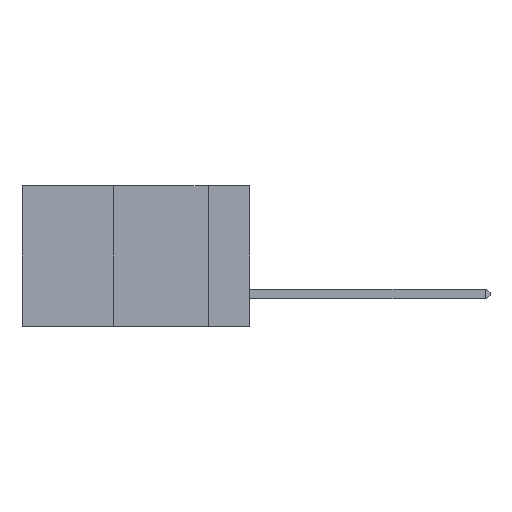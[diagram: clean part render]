
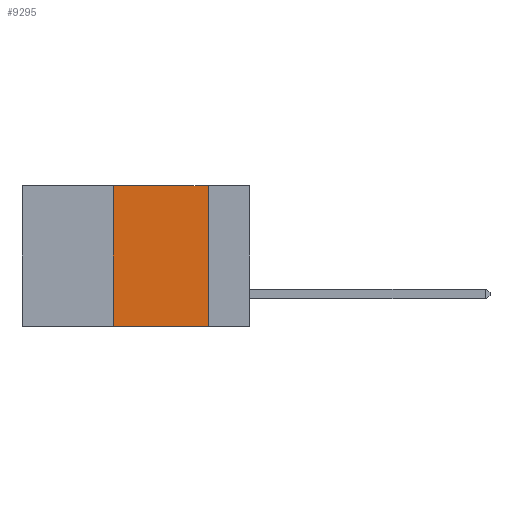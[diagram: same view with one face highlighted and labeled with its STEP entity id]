
A CAD part, left-side view. The second image highlights one B-rep face of the part: STEP entity #9295.
In plain terms, the highlighted planar face has unit normal (-1, 0, 0).
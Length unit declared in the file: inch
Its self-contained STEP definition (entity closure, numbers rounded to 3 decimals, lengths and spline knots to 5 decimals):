
#274 = ORIENTED_EDGE ( 'NONE', *, *, #9508, .F. ) ;
#290 = ORIENTED_EDGE ( 'NONE', *, *, #12163, .F. ) ;
#353 = ORIENTED_EDGE ( 'NONE', *, *, #3737, .F. ) ;
#403 = LINE ( 'NONE', #6212, #2656 ) ;
#404 = ORIENTED_EDGE ( 'NONE', *, *, #12074, .T. ) ;
#520 = LINE ( 'NONE', #2945, #10806 ) ;
#1215 = AXIS2_PLACEMENT_3D ( 'NONE', #3625, #4772, #11905 ) ;
#1304 = VERTEX_POINT ( 'NONE', #1729 ) ;
#1729 = CARTESIAN_POINT ( 'NONE',  ( 0., 0.36, -0.37 ) ) ;
#1730 = LINE ( 'NONE', #8205, #6918 ) ;
#2656 = VECTOR ( 'NONE', #5117, 39.37008 ) ;
#2933 = VECTOR ( 'NONE', #11274, 39.37008 ) ;
#2945 = CARTESIAN_POINT ( 'NONE',  ( 0., 0.36, 0. ) ) ;
#3074 = VERTEX_POINT ( 'NONE', #5282 ) ;
#3278 = LINE ( 'NONE', #10295, #2933 ) ;
#3625 = CARTESIAN_POINT ( 'NONE',  ( 0., 0.6, 0. ) ) ;
#3737 = EDGE_CURVE ( 'NONE', #1304, #3074, #520, .T. ) ;
#4772 = DIRECTION ( 'NONE',  ( 1., 0., 0. ) ) ;
#5117 = DIRECTION ( 'NONE',  ( 0., 0., -1. ) ) ;
#5282 = CARTESIAN_POINT ( 'NONE',  ( 0., 0.36, 0. ) ) ;
#6144 = DIRECTION ( 'NONE',  ( 0., -1., 0. ) ) ;
#6212 = CARTESIAN_POINT ( 'NONE',  ( 0., 0.11, 0. ) ) ;
#6918 = VECTOR ( 'NONE', #6144, 39.37008 ) ;
#7925 = CARTESIAN_POINT ( 'NONE',  ( 0., 0.11, 0. ) ) ;
#8205 = CARTESIAN_POINT ( 'NONE',  ( 0., 0.6, -0.37 ) ) ;
#9295 = ADVANCED_FACE ( 'NONE', ( #13478 ), #9951, .F. ) ;
#9508 = EDGE_CURVE ( 'NONE', #11434, #10222, #403, .T. ) ;
#9951 = PLANE ( 'NONE',  #1215 ) ;
#10222 = VERTEX_POINT ( 'NONE', #10843 ) ;
#10295 = CARTESIAN_POINT ( 'NONE',  ( 0., 0.6, 0. ) ) ;
#10358 = DIRECTION ( 'NONE',  ( 0., 0., 1. ) ) ;
#10806 = VECTOR ( 'NONE', #10358, 39.37008 ) ;
#10843 = CARTESIAN_POINT ( 'NONE',  ( 0., 0.11, -0.37 ) ) ;
#11274 = DIRECTION ( 'NONE',  ( 0., -1., 0. ) ) ;
#11434 = VERTEX_POINT ( 'NONE', #7925 ) ;
#11905 = DIRECTION ( 'NONE',  ( 0., 0., -1. ) ) ;
#12074 = EDGE_CURVE ( 'NONE', #1304, #10222, #1730, .T. ) ;
#12163 = EDGE_CURVE ( 'NONE', #3074, #11434, #3278, .T. ) ;
#12233 = EDGE_LOOP ( 'NONE', ( #274, #290, #353, #404 ) ) ;
#13478 = FACE_OUTER_BOUND ( 'NONE', #12233, .T. ) ;
